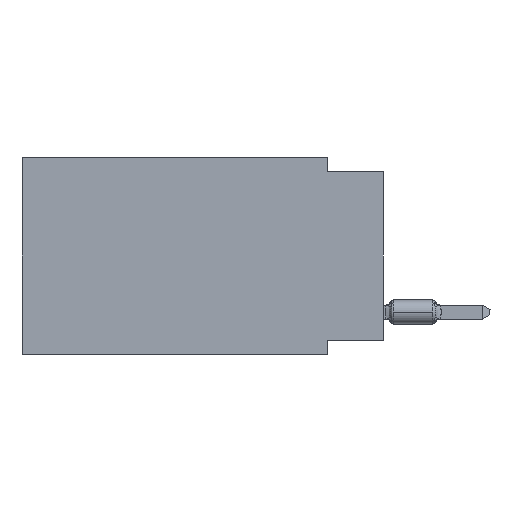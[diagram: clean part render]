
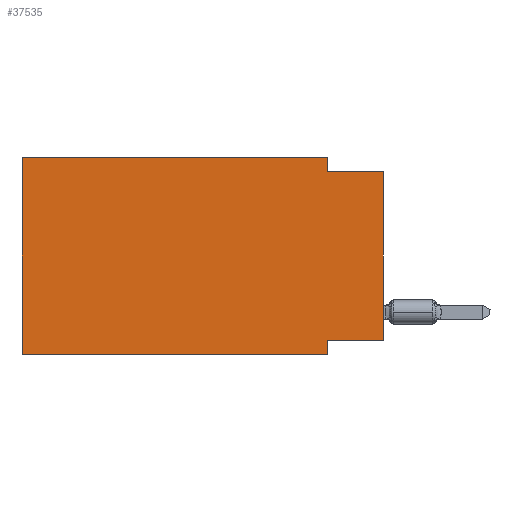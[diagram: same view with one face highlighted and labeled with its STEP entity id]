
A CAD part, left-side view. The second image highlights one B-rep face of the part: STEP entity #37535.
In plain terms, the highlighted planar face has unit normal (-1, 0, 0).
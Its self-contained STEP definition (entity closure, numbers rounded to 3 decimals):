
#1313 = DIRECTION ( 'NONE',  ( 0., 0., -1. ) ) ;
#3061 = ORIENTED_EDGE ( 'NONE', *, *, #26158, .T. ) ;
#3435 = VERTEX_POINT ( 'NONE', #4546 ) ;
#4546 = CARTESIAN_POINT ( 'NONE',  ( 0., 2.54, -0.635 ) ) ;
#5109 = DIRECTION ( 'NONE',  ( 0., 0., 1. ) ) ;
#5614 = CARTESIAN_POINT ( 'NONE',  ( 0., 16.383, -8.89 ) ) ;
#5693 = CARTESIAN_POINT ( 'NONE',  ( 0., 16.383, -8.89 ) ) ;
#5891 = CARTESIAN_POINT ( 'NONE',  ( 0., 2.54, -8.89 ) ) ;
#6423 = VERTEX_POINT ( 'NONE', #63990 ) ;
#6645 = VECTOR ( 'NONE', #1313, 1000. ) ;
#7381 = EDGE_CURVE ( 'NONE', #57493, #63246, #72125, .T. ) ;
#7468 = CARTESIAN_POINT ( 'NONE',  ( 0., 2.54, -8.255 ) ) ;
#7477 = EDGE_CURVE ( 'NONE', #25126, #40957, #34131, .T. ) ;
#8522 = CARTESIAN_POINT ( 'NONE',  ( 0., 16.383, 0. ) ) ;
#9894 = CARTESIAN_POINT ( 'NONE',  ( 0., 0., 0. ) ) ;
#11777 = VECTOR ( 'NONE', #27938, 1000. ) ;
#13094 = VECTOR ( 'NONE', #42139, 1000. ) ;
#13908 = CARTESIAN_POINT ( 'NONE',  ( 0., 16.383, 0. ) ) ;
#14133 = VECTOR ( 'NONE', #56783, 1000. ) ;
#14773 = CARTESIAN_POINT ( 'NONE',  ( 0., 16.383, 0. ) ) ;
#16186 = EDGE_CURVE ( 'NONE', #3435, #6423, #45589, .T. ) ;
#16882 = DIRECTION ( 'NONE',  ( 0., 0., -1. ) ) ;
#16924 = EDGE_CURVE ( 'NONE', #25126, #20426, #69228, .T. ) ;
#17099 = PLANE ( 'NONE',  #64644 ) ;
#20426 = VERTEX_POINT ( 'NONE', #13908 ) ;
#21496 = DIRECTION ( 'NONE',  ( 1., 0., 0. ) ) ;
#23146 = CARTESIAN_POINT ( 'NONE',  ( 0., 0., -8.255 ) ) ;
#23611 = LINE ( 'NONE', #50263, #6645 ) ;
#24137 = ORIENTED_EDGE ( 'NONE', *, *, #30078, .F. ) ;
#25011 = LINE ( 'NONE', #8522, #13094 ) ;
#25126 = VERTEX_POINT ( 'NONE', #5693 ) ;
#26158 = EDGE_CURVE ( 'NONE', #57493, #6423, #49687, .T. ) ;
#27338 = CARTESIAN_POINT ( 'NONE',  ( 0., 16.383, 0. ) ) ;
#27938 = DIRECTION ( 'NONE',  ( 0., -1., 0. ) ) ;
#29547 = EDGE_LOOP ( 'NONE', ( #3061, #56665, #68972, #24137, #65100, #67024, #41772, #58311 ) ) ;
#30078 = EDGE_CURVE ( 'NONE', #20426, #37681, #25011, .T. ) ;
#34131 = LINE ( 'NONE', #5614, #11777 ) ;
#37535 = ADVANCED_FACE ( 'NONE', ( #39375 ), #17099, .F. ) ;
#37681 = VERTEX_POINT ( 'NONE', #38295 ) ;
#38278 = CARTESIAN_POINT ( 'NONE',  ( 0., 2.54, -8.89 ) ) ;
#38295 = CARTESIAN_POINT ( 'NONE',  ( 0., 2.54, 0. ) ) ;
#39375 = FACE_OUTER_BOUND ( 'NONE', #29547, .T. ) ;
#40481 = CARTESIAN_POINT ( 'NONE',  ( 0., 0., -0.635 ) ) ;
#40621 = VECTOR ( 'NONE', #5109, 1000. ) ;
#40957 = VERTEX_POINT ( 'NONE', #38278 ) ;
#41772 = ORIENTED_EDGE ( 'NONE', *, *, #44128, .F. ) ;
#42139 = DIRECTION ( 'NONE',  ( 0., -1., 0. ) ) ;
#43203 = LINE ( 'NONE', #5891, #61386 ) ;
#43401 = DIRECTION ( 'NONE',  ( 0., 0., -1. ) ) ;
#43879 = DIRECTION ( 'NONE',  ( 0., -1., 0. ) ) ;
#44128 = EDGE_CURVE ( 'NONE', #63246, #40957, #43203, .T. ) ;
#45589 = LINE ( 'NONE', #40481, #65495 ) ;
#49687 = LINE ( 'NONE', #9894, #40621 ) ;
#50020 = EDGE_CURVE ( 'NONE', #37681, #3435, #23611, .T. ) ;
#50263 = CARTESIAN_POINT ( 'NONE',  ( 0., 2.54, 0. ) ) ;
#56665 = ORIENTED_EDGE ( 'NONE', *, *, #16186, .F. ) ;
#56783 = DIRECTION ( 'NONE',  ( 0., 1., 0. ) ) ;
#57493 = VERTEX_POINT ( 'NONE', #23146 ) ;
#58311 = ORIENTED_EDGE ( 'NONE', *, *, #7381, .F. ) ;
#61386 = VECTOR ( 'NONE', #16882, 1000. ) ;
#61899 = CARTESIAN_POINT ( 'NONE',  ( 0., 0., -8.255 ) ) ;
#63246 = VERTEX_POINT ( 'NONE', #7468 ) ;
#63990 = CARTESIAN_POINT ( 'NONE',  ( 0., 0., -0.635 ) ) ;
#64464 = VECTOR ( 'NONE', #70288, 1000. ) ;
#64644 = AXIS2_PLACEMENT_3D ( 'NONE', #27338, #21496, #43401 ) ;
#65100 = ORIENTED_EDGE ( 'NONE', *, *, #16924, .F. ) ;
#65495 = VECTOR ( 'NONE', #43879, 1000. ) ;
#67024 = ORIENTED_EDGE ( 'NONE', *, *, #7477, .T. ) ;
#68972 = ORIENTED_EDGE ( 'NONE', *, *, #50020, .F. ) ;
#69228 = LINE ( 'NONE', #14773, #64464 ) ;
#70288 = DIRECTION ( 'NONE',  ( 0., 0., 1. ) ) ;
#72125 = LINE ( 'NONE', #61899, #14133 ) ;
